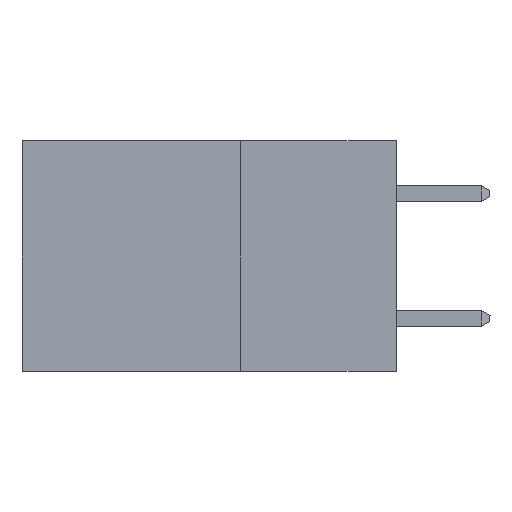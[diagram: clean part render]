
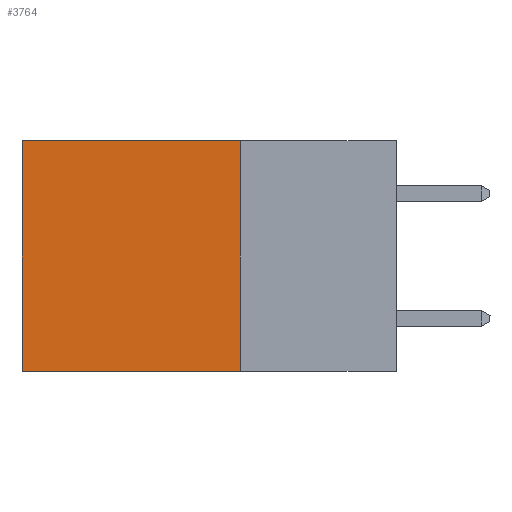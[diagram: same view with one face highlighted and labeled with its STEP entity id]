
A CAD part, left-side view. The second image highlights one B-rep face of the part: STEP entity #3764.
In plain terms, the highlighted planar face has unit normal (-1, 0, 0).
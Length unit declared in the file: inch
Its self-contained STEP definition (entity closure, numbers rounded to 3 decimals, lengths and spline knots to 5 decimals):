
#990 = CARTESIAN_POINT ( 'NONE',  ( 0.2615, 0.6, 0. ) ) ;
#1187 = VERTEX_POINT ( 'NONE', #6132 ) ;
#1646 = EDGE_LOOP ( 'NONE', ( #4955, #5098, #5110, #5259 ) ) ;
#2040 = VERTEX_POINT ( 'NONE', #990 ) ;
#2189 = EDGE_CURVE ( 'NONE', #2040, #1187, #9883, .T. ) ;
#2372 = EDGE_CURVE ( 'NONE', #7261, #1187, #4853, .T. ) ;
#2439 = VECTOR ( 'NONE', #7682, 39.37008 ) ;
#3162 = LINE ( 'NONE', #7989, #9115 ) ;
#3673 = CARTESIAN_POINT ( 'NONE',  ( 0.2615, 0.6, -0.37 ) ) ;
#3764 = ADVANCED_FACE ( 'NONE', ( #8791 ), #7714, .F. ) ;
#4155 = LINE ( 'NONE', #4399, #9841 ) ;
#4293 = EDGE_CURVE ( 'NONE', #10109, #7261, #4155, .T. ) ;
#4324 = DIRECTION ( 'NONE',  ( 0., 0., -1. ) ) ;
#4399 = CARTESIAN_POINT ( 'NONE',  ( 0.2615, 0.25, -0.37 ) ) ;
#4568 = DIRECTION ( 'NONE',  ( 0., 0., -1. ) ) ;
#4853 = LINE ( 'NONE', #8364, #2439 ) ;
#4858 = DIRECTION ( 'NONE',  ( 0., 1., 0. ) ) ;
#4955 = ORIENTED_EDGE ( 'NONE', *, *, #2189, .T. ) ;
#5098 = ORIENTED_EDGE ( 'NONE', *, *, #2372, .F. ) ;
#5110 = ORIENTED_EDGE ( 'NONE', *, *, #4293, .F. ) ;
#5259 = ORIENTED_EDGE ( 'NONE', *, *, #9716, .T. ) ;
#5833 = VECTOR ( 'NONE', #4568, 39.37008 ) ;
#6132 = CARTESIAN_POINT ( 'NONE',  ( 0.2615, 0.6, -0.37 ) ) ;
#6922 = CARTESIAN_POINT ( 'NONE',  ( 0.2615, 0.25, 0. ) ) ;
#7261 = VERTEX_POINT ( 'NONE', #7409 ) ;
#7409 = CARTESIAN_POINT ( 'NONE',  ( 0.2615, 0.25, -0.37 ) ) ;
#7670 = DIRECTION ( 'NONE',  ( 0., 0., -1. ) ) ;
#7682 = DIRECTION ( 'NONE',  ( 0., 1., 0. ) ) ;
#7693 = DIRECTION ( 'NONE',  ( 1., 0., 0. ) ) ;
#7711 = CARTESIAN_POINT ( 'NONE',  ( 0.2615, 0.25, -0.37 ) ) ;
#7714 = PLANE ( 'NONE',  #8677 ) ;
#7989 = CARTESIAN_POINT ( 'NONE',  ( 0.2615, 0.25, 0. ) ) ;
#8364 = CARTESIAN_POINT ( 'NONE',  ( 0.2615, 0.25, -0.37 ) ) ;
#8677 = AXIS2_PLACEMENT_3D ( 'NONE', #7711, #7693, #7670 ) ;
#8791 = FACE_OUTER_BOUND ( 'NONE', #1646, .T. ) ;
#9115 = VECTOR ( 'NONE', #4858, 39.37008 ) ;
#9716 = EDGE_CURVE ( 'NONE', #10109, #2040, #3162, .T. ) ;
#9841 = VECTOR ( 'NONE', #4324, 39.37008 ) ;
#9883 = LINE ( 'NONE', #3673, #5833 ) ;
#10109 = VERTEX_POINT ( 'NONE', #6922 ) ;
